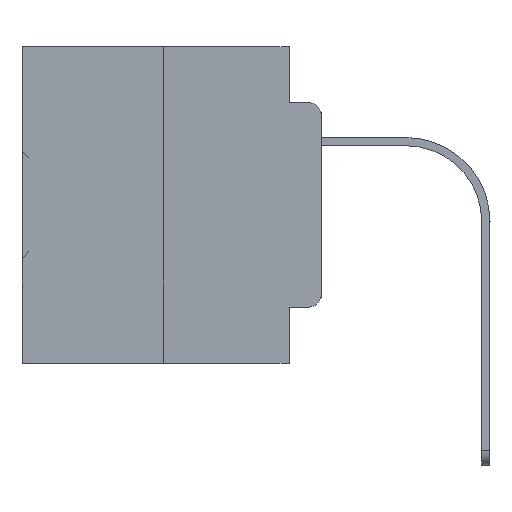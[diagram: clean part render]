
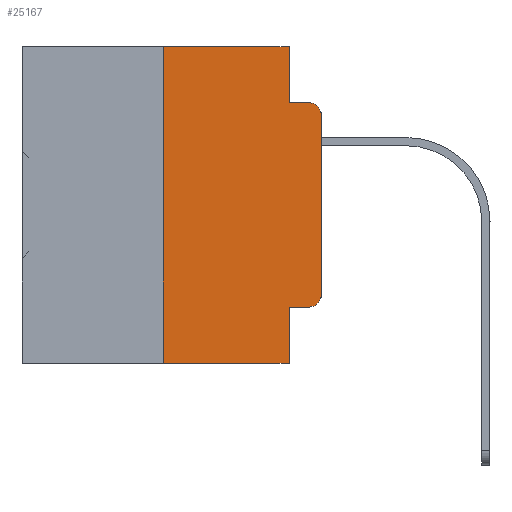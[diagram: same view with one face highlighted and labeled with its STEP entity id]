
A CAD part, left-side view. The second image highlights one B-rep face of the part: STEP entity #25167.
In plain terms, the highlighted planar face has unit normal (-1, 0, 0).
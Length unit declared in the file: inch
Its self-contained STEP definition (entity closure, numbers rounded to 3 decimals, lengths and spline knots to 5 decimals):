
#351 = CARTESIAN_POINT ( 'NONE',  ( 0., 0.25, -0.5 ) ) ;
#506 = DIRECTION ( 'NONE',  ( 0., 0., -1. ) ) ;
#706 = CARTESIAN_POINT ( 'NONE',  ( 0., 0., -0.1085 ) ) ;
#890 = EDGE_CURVE ( 'NONE', #29283, #26321, #10225, .T. ) ;
#2354 = AXIS2_PLACEMENT_3D ( 'NONE', #7293, #6927, #18780 ) ;
#2917 = EDGE_CURVE ( 'NONE', #11120, #28222, #18595, .T. ) ;
#2970 = AXIS2_PLACEMENT_3D ( 'NONE', #7933, #33948, #27898 ) ;
#3852 = VECTOR ( 'NONE', #30041, 39.37008 ) ;
#4231 = DIRECTION ( 'NONE',  ( 0., -1., 0. ) ) ;
#4637 = DIRECTION ( 'NONE',  ( 0., 0., 1. ) ) ;
#4710 = CARTESIAN_POINT ( 'NONE',  ( 0., 0.051, -0.0885 ) ) ;
#4756 = DIRECTION ( 'NONE',  ( 0., 0., -1. ) ) ;
#4847 = VECTOR ( 'NONE', #4637, 39.37008 ) ;
#5119 = ORIENTED_EDGE ( 'NONE', *, *, #34914, .F. ) ;
#5868 = DIRECTION ( 'NONE',  ( 0., 0., 1. ) ) ;
#6543 = LINE ( 'NONE', #17301, #28996 ) ;
#6637 = VERTEX_POINT ( 'NONE', #12925 ) ;
#6927 = DIRECTION ( 'NONE',  ( -1., 0., 0. ) ) ;
#6980 = DIRECTION ( 'NONE',  ( 0., 0., -1. ) ) ;
#7075 = LINE ( 'NONE', #18551, #3852 ) ;
#7293 = CARTESIAN_POINT ( 'NONE',  ( 0., 0.02, -0.3915 ) ) ;
#7779 = CARTESIAN_POINT ( 'NONE',  ( 0., 0.25, 0. ) ) ;
#7933 = CARTESIAN_POINT ( 'NONE',  ( 0., 0.02, -0.1085 ) ) ;
#8323 = DIRECTION ( 'NONE',  ( 0., -1., 0. ) ) ;
#9100 = ORIENTED_EDGE ( 'NONE', *, *, #890, .T. ) ;
#10095 = ORIENTED_EDGE ( 'NONE', *, *, #34911, .F. ) ;
#10225 = CIRCLE ( 'NONE', #2970, 0.02 ) ;
#10557 = ORIENTED_EDGE ( 'NONE', *, *, #2917, .T. ) ;
#10727 = ORIENTED_EDGE ( 'NONE', *, *, #28609, .T. ) ;
#11120 = VERTEX_POINT ( 'NONE', #27444 ) ;
#12047 = CARTESIAN_POINT ( 'NONE',  ( 0., 0.051, 0. ) ) ;
#12062 = LINE ( 'NONE', #20372, #32472 ) ;
#12925 = CARTESIAN_POINT ( 'NONE',  ( 0., 0.051, -0.4115 ) ) ;
#13046 = ORIENTED_EDGE ( 'NONE', *, *, #22748, .F. ) ;
#13056 = CARTESIAN_POINT ( 'NONE',  ( 0., 0.02, -0.0885 ) ) ;
#13360 = DIRECTION ( 'NONE',  ( 0., -1., 0. ) ) ;
#13766 = EDGE_LOOP ( 'NONE', ( #31512, #9100, #5119, #13046, #24803, #33633, #10727, #10095, #36501, #10557 ) ) ;
#16476 = VECTOR ( 'NONE', #13360, 39.37008 ) ;
#17301 = CARTESIAN_POINT ( 'NONE',  ( 0., 0.051, 0. ) ) ;
#18551 = CARTESIAN_POINT ( 'NONE',  ( 0., 0.051, -0.4115 ) ) ;
#18575 = VECTOR ( 'NONE', #8323, 39.37008 ) ;
#18595 = CIRCLE ( 'NONE', #2354, 0.02 ) ;
#18780 = DIRECTION ( 'NONE',  ( 0., 0., -1. ) ) ;
#19521 = CARTESIAN_POINT ( 'NONE',  ( 0., 0.051, -0.5 ) ) ;
#19883 = EDGE_CURVE ( 'NONE', #28222, #29283, #30652, .T. ) ;
#20372 = CARTESIAN_POINT ( 'NONE',  ( 0., 0.25, 0. ) ) ;
#21027 = VERTEX_POINT ( 'NONE', #12047 ) ;
#21670 = VECTOR ( 'NONE', #4231, 39.37008 ) ;
#22279 = CARTESIAN_POINT ( 'NONE',  ( 0., 0.473, 0. ) ) ;
#22748 = EDGE_CURVE ( 'NONE', #21027, #25634, #6543, .T. ) ;
#24595 = CARTESIAN_POINT ( 'NONE',  ( 0., 0., 0. ) ) ;
#24803 = ORIENTED_EDGE ( 'NONE', *, *, #27421, .F. ) ;
#24821 = CARTESIAN_POINT ( 'NONE',  ( 0., 0., -0.3915 ) ) ;
#25096 = PLANE ( 'NONE',  #25528 ) ;
#25167 = ADVANCED_FACE ( 'NONE', ( #33600 ), #25096, .F. ) ;
#25528 = AXIS2_PLACEMENT_3D ( 'NONE', #22279, #33787, #4756 ) ;
#25634 = VERTEX_POINT ( 'NONE', #4710 ) ;
#26321 = VERTEX_POINT ( 'NONE', #13056 ) ;
#27090 = CARTESIAN_POINT ( 'NONE',  ( 0., 0.051, 0. ) ) ;
#27216 = CARTESIAN_POINT ( 'NONE',  ( 0., 0.473, -0.5 ) ) ;
#27391 = VERTEX_POINT ( 'NONE', #7779 ) ;
#27421 = EDGE_CURVE ( 'NONE', #27391, #21027, #30972, .T. ) ;
#27444 = CARTESIAN_POINT ( 'NONE',  ( 0., 0.02, -0.4115 ) ) ;
#27496 = EDGE_CURVE ( 'NONE', #28008, #27391, #12062, .T. ) ;
#27898 = DIRECTION ( 'NONE',  ( 0., 0., -1. ) ) ;
#28008 = VERTEX_POINT ( 'NONE', #351 ) ;
#28222 = VERTEX_POINT ( 'NONE', #24821 ) ;
#28609 = EDGE_CURVE ( 'NONE', #28008, #28741, #33471, .T. ) ;
#28741 = VERTEX_POINT ( 'NONE', #19521 ) ;
#28996 = VECTOR ( 'NONE', #506, 39.37008 ) ;
#29283 = VERTEX_POINT ( 'NONE', #706 ) ;
#29707 = VECTOR ( 'NONE', #6980, 39.37008 ) ;
#30041 = DIRECTION ( 'NONE',  ( 0., -1., 0. ) ) ;
#30127 = CARTESIAN_POINT ( 'NONE',  ( 0., 0.051, -0.0885 ) ) ;
#30652 = LINE ( 'NONE', #24595, #4847 ) ;
#30972 = LINE ( 'NONE', #35737, #18575 ) ;
#31512 = ORIENTED_EDGE ( 'NONE', *, *, #19883, .T. ) ;
#32472 = VECTOR ( 'NONE', #5868, 39.37008 ) ;
#33471 = LINE ( 'NONE', #27216, #21670 ) ;
#33544 = LINE ( 'NONE', #30127, #16476 ) ;
#33600 = FACE_OUTER_BOUND ( 'NONE', #13766, .T. ) ;
#33633 = ORIENTED_EDGE ( 'NONE', *, *, #27496, .F. ) ;
#33787 = DIRECTION ( 'NONE',  ( 1., 0., 0. ) ) ;
#33948 = DIRECTION ( 'NONE',  ( -1., 0., 0. ) ) ;
#34911 = EDGE_CURVE ( 'NONE', #6637, #28741, #36179, .T. ) ;
#34914 = EDGE_CURVE ( 'NONE', #25634, #26321, #33544, .T. ) ;
#35293 = EDGE_CURVE ( 'NONE', #6637, #11120, #7075, .T. ) ;
#35737 = CARTESIAN_POINT ( 'NONE',  ( 0., 0.473, 0. ) ) ;
#36179 = LINE ( 'NONE', #27090, #29707 ) ;
#36501 = ORIENTED_EDGE ( 'NONE', *, *, #35293, .T. ) ;
